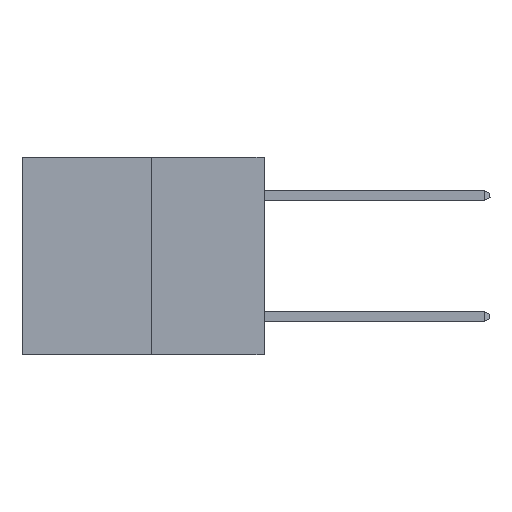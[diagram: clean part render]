
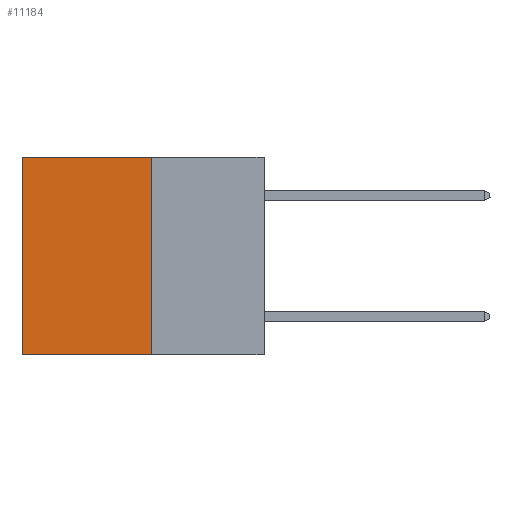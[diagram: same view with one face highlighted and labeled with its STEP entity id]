
A CAD part, left-side view. The second image highlights one B-rep face of the part: STEP entity #11184.
In plain terms, the highlighted planar face has unit normal (-1, 0, 0).
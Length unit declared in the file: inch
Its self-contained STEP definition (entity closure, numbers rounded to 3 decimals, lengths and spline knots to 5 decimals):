
#819 = DIRECTION ( 'NONE',  ( 0., 1., 0. ) ) ;
#1639 = EDGE_CURVE ( 'NONE', #28052, #12177, #8539, .T. ) ;
#2836 = CARTESIAN_POINT ( 'NONE',  ( 0.3165, 0.6, -0.49 ) ) ;
#3164 = ORIENTED_EDGE ( 'NONE', *, *, #10229, .F. ) ;
#4879 = CARTESIAN_POINT ( 'NONE',  ( 0.3165, 0.6, 0. ) ) ;
#6876 = VERTEX_POINT ( 'NONE', #11790 ) ;
#7469 = AXIS2_PLACEMENT_3D ( 'NONE', #18818, #7879, #15461 ) ;
#7879 = DIRECTION ( 'NONE',  ( 1., 0., 0. ) ) ;
#8539 = LINE ( 'NONE', #17175, #12987 ) ;
#9423 = CARTESIAN_POINT ( 'NONE',  ( 0.3165, 0.28, -0.49 ) ) ;
#10229 = EDGE_CURVE ( 'NONE', #6876, #27945, #14895, .T. ) ;
#10526 = LINE ( 'NONE', #14242, #15002 ) ;
#11008 = DIRECTION ( 'NONE',  ( 0., 0., -1. ) ) ;
#11184 = ADVANCED_FACE ( 'NONE', ( #16531 ), #27115, .F. ) ;
#11669 = CARTESIAN_POINT ( 'NONE',  ( 0.3165, 0.28, 0. ) ) ;
#11790 = CARTESIAN_POINT ( 'NONE',  ( 0.3165, 0.28, -0.49 ) ) ;
#12177 = VERTEX_POINT ( 'NONE', #4879 ) ;
#12987 = VECTOR ( 'NONE', #17081, 39.37008 ) ;
#14242 = CARTESIAN_POINT ( 'NONE',  ( 0.3165, 0.6, -0.49 ) ) ;
#14499 = ORIENTED_EDGE ( 'NONE', *, *, #1639, .T. ) ;
#14895 = LINE ( 'NONE', #9423, #17920 ) ;
#15002 = VECTOR ( 'NONE', #22953, 39.37008 ) ;
#15461 = DIRECTION ( 'NONE',  ( 0., 0., -1. ) ) ;
#15596 = ORIENTED_EDGE ( 'NONE', *, *, #27931, .F. ) ;
#16531 = FACE_OUTER_BOUND ( 'NONE', #26931, .T. ) ;
#17081 = DIRECTION ( 'NONE',  ( 0., 1., 0. ) ) ;
#17175 = CARTESIAN_POINT ( 'NONE',  ( 0.3165, 0.28, 0. ) ) ;
#17920 = VECTOR ( 'NONE', #819, 39.37008 ) ;
#18818 = CARTESIAN_POINT ( 'NONE',  ( 0.3165, 0.28, -0.49 ) ) ;
#19286 = VECTOR ( 'NONE', #11008, 39.37008 ) ;
#20794 = EDGE_CURVE ( 'NONE', #12177, #27945, #10526, .T. ) ;
#21934 = CARTESIAN_POINT ( 'NONE',  ( 0.3165, 0.28, -0.49 ) ) ;
#22255 = ORIENTED_EDGE ( 'NONE', *, *, #20794, .T. ) ;
#22953 = DIRECTION ( 'NONE',  ( 0., 0., -1. ) ) ;
#24350 = LINE ( 'NONE', #21934, #19286 ) ;
#26931 = EDGE_LOOP ( 'NONE', ( #22255, #3164, #15596, #14499 ) ) ;
#27115 = PLANE ( 'NONE',  #7469 ) ;
#27931 = EDGE_CURVE ( 'NONE', #28052, #6876, #24350, .T. ) ;
#27945 = VERTEX_POINT ( 'NONE', #2836 ) ;
#28052 = VERTEX_POINT ( 'NONE', #11669 ) ;
